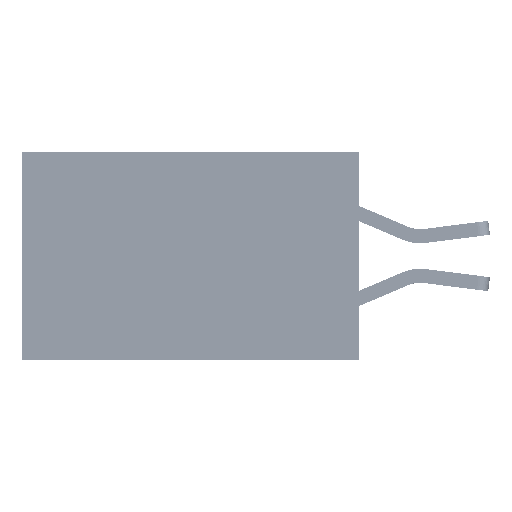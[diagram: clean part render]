
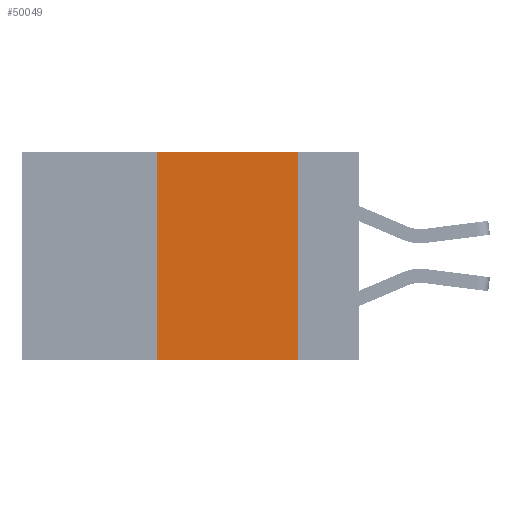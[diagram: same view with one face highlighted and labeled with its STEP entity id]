
A CAD part, left-side view. The second image highlights one B-rep face of the part: STEP entity #50049.
In plain terms, the highlighted planar face has unit normal (-1, 0, 0).
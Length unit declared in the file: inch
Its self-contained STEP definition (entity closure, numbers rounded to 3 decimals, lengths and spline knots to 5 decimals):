
#538 = VECTOR ( 'NONE', #13878, 39.37008 ) ;
#1396 = EDGE_CURVE ( 'NONE', #36453, #11787, #38996, .T. ) ;
#1701 = LINE ( 'NONE', #33961, #20662 ) ;
#7504 = DIRECTION ( 'NONE',  ( 0., 0., 1. ) ) ;
#7883 = CARTESIAN_POINT ( 'NONE',  ( 0., 0.36, 0. ) ) ;
#8499 = LINE ( 'NONE', #35957, #41967 ) ;
#10613 = EDGE_CURVE ( 'NONE', #36453, #13114, #46634, .T. ) ;
#10677 = ORIENTED_EDGE ( 'NONE', *, *, #10613, .F. ) ;
#11787 = VERTEX_POINT ( 'NONE', #27901 ) ;
#13114 = VERTEX_POINT ( 'NONE', #7883 ) ;
#13878 = DIRECTION ( 'NONE',  ( 0., -1., 0. ) ) ;
#14119 = ORIENTED_EDGE ( 'NONE', *, *, #47835, .F. ) ;
#15522 = DIRECTION ( 'NONE',  ( 0., -1., 0. ) ) ;
#15595 = DIRECTION ( 'NONE',  ( 0., 0., -1. ) ) ;
#18506 = FACE_OUTER_BOUND ( 'NONE', #20408, .T. ) ;
#20408 = EDGE_LOOP ( 'NONE', ( #14119, #35962, #10677, #34163 ) ) ;
#20662 = VECTOR ( 'NONE', #25518, 39.37008 ) ;
#23927 = DIRECTION ( 'NONE',  ( 1., 0., 0. ) ) ;
#25518 = DIRECTION ( 'NONE',  ( 0., 0., -1. ) ) ;
#25813 = CARTESIAN_POINT ( 'NONE',  ( 0., 0.11, 0. ) ) ;
#26409 = CARTESIAN_POINT ( 'NONE',  ( 0., 0.6, -0.37 ) ) ;
#27228 = VERTEX_POINT ( 'NONE', #25813 ) ;
#27901 = CARTESIAN_POINT ( 'NONE',  ( 0., 0.11, -0.37 ) ) ;
#29353 = EDGE_CURVE ( 'NONE', #13114, #27228, #8499, .T. ) ;
#30750 = AXIS2_PLACEMENT_3D ( 'NONE', #48407, #23927, #15595 ) ;
#33961 = CARTESIAN_POINT ( 'NONE',  ( 0., 0.11, 0. ) ) ;
#34163 = ORIENTED_EDGE ( 'NONE', *, *, #1396, .T. ) ;
#35957 = CARTESIAN_POINT ( 'NONE',  ( 0., 0.6, 0. ) ) ;
#35962 = ORIENTED_EDGE ( 'NONE', *, *, #29353, .F. ) ;
#36453 = VERTEX_POINT ( 'NONE', #43022 ) ;
#38996 = LINE ( 'NONE', #26409, #538 ) ;
#41967 = VECTOR ( 'NONE', #15522, 39.37008 ) ;
#43022 = CARTESIAN_POINT ( 'NONE',  ( 0., 0.36, -0.37 ) ) ;
#46634 = LINE ( 'NONE', #52182, #49775 ) ;
#47835 = EDGE_CURVE ( 'NONE', #27228, #11787, #1701, .T. ) ;
#48221 = PLANE ( 'NONE',  #30750 ) ;
#48407 = CARTESIAN_POINT ( 'NONE',  ( 0., 0.6, 0. ) ) ;
#49775 = VECTOR ( 'NONE', #7504, 39.37008 ) ;
#50049 = ADVANCED_FACE ( 'NONE', ( #18506 ), #48221, .F. ) ;
#52182 = CARTESIAN_POINT ( 'NONE',  ( 0., 0.36, 0. ) ) ;
